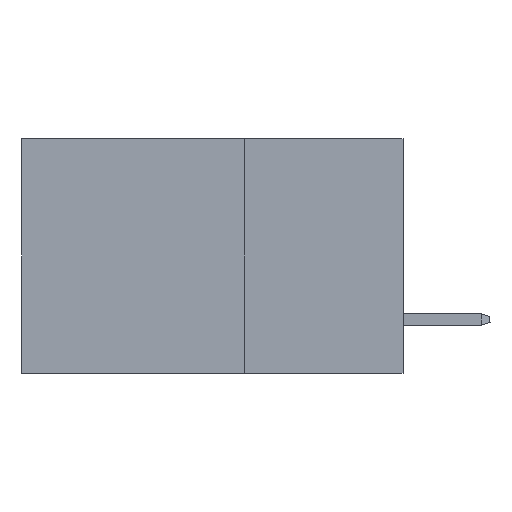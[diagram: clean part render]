
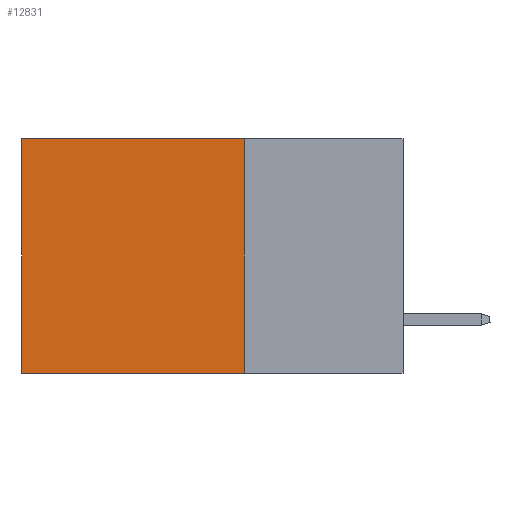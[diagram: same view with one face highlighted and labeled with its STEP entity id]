
A CAD part, left-side view. The second image highlights one B-rep face of the part: STEP entity #12831.
In plain terms, the highlighted planar face has unit normal (-1, 0, 0).
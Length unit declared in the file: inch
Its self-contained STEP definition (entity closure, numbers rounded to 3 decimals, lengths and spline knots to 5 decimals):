
#256 = VERTEX_POINT ( 'NONE', #8918 ) ;
#1142 = CARTESIAN_POINT ( 'NONE',  ( 0.2875, 0.25, -0.37 ) ) ;
#1535 = CARTESIAN_POINT ( 'NONE',  ( 0.2875, 0.25, 0. ) ) ;
#1874 = LINE ( 'NONE', #1535, #11847 ) ;
#2513 = CARTESIAN_POINT ( 'NONE',  ( 0.2875, 0.25, 0. ) ) ;
#3116 = EDGE_CURVE ( 'NONE', #13336, #14258, #14459, .T. ) ;
#3217 = VERTEX_POINT ( 'NONE', #13743 ) ;
#3584 = ORIENTED_EDGE ( 'NONE', *, *, #3116, .F. ) ;
#3779 = CARTESIAN_POINT ( 'NONE',  ( 0.2875, 0.25, 0. ) ) ;
#4141 = CARTESIAN_POINT ( 'NONE',  ( 0.2875, 0.6, 0. ) ) ;
#4988 = VECTOR ( 'NONE', #9345, 39.37008 ) ;
#6195 = DIRECTION ( 'NONE',  ( 0., 1., 0. ) ) ;
#7062 = EDGE_CURVE ( 'NONE', #3217, #14258, #15848, .T. ) ;
#7212 = ORIENTED_EDGE ( 'NONE', *, *, #7062, .T. ) ;
#8063 = EDGE_CURVE ( 'NONE', #256, #3217, #9187, .T. ) ;
#8296 = EDGE_LOOP ( 'NONE', ( #7212, #3584, #14886, #15418 ) ) ;
#8822 = FACE_OUTER_BOUND ( 'NONE', #8296, .T. ) ;
#8918 = CARTESIAN_POINT ( 'NONE',  ( 0.2875, 0.25, 0. ) ) ;
#9187 = LINE ( 'NONE', #2513, #16423 ) ;
#9327 = EDGE_CURVE ( 'NONE', #256, #13336, #1874, .T. ) ;
#9345 = DIRECTION ( 'NONE',  ( 0., 0., -1. ) ) ;
#9765 = CARTESIAN_POINT ( 'NONE',  ( 0.2875, 0.6, -0.37 ) ) ;
#10184 = DIRECTION ( 'NONE',  ( 1., 0., 0. ) ) ;
#11100 = CARTESIAN_POINT ( 'NONE',  ( 0.2875, 0.25, -0.37 ) ) ;
#11428 = VECTOR ( 'NONE', #15500, 39.37008 ) ;
#11847 = VECTOR ( 'NONE', #12195, 39.37008 ) ;
#12195 = DIRECTION ( 'NONE',  ( 0., 0., -1. ) ) ;
#12831 = ADVANCED_FACE ( 'NONE', ( #8822 ), #16748, .F. ) ;
#13008 = AXIS2_PLACEMENT_3D ( 'NONE', #3779, #10184, #16655 ) ;
#13336 = VERTEX_POINT ( 'NONE', #11100 ) ;
#13743 = CARTESIAN_POINT ( 'NONE',  ( 0.2875, 0.6, 0. ) ) ;
#14258 = VERTEX_POINT ( 'NONE', #9765 ) ;
#14459 = LINE ( 'NONE', #1142, #11428 ) ;
#14886 = ORIENTED_EDGE ( 'NONE', *, *, #9327, .F. ) ;
#15418 = ORIENTED_EDGE ( 'NONE', *, *, #8063, .T. ) ;
#15500 = DIRECTION ( 'NONE',  ( 0., 1., 0. ) ) ;
#15848 = LINE ( 'NONE', #4141, #4988 ) ;
#16423 = VECTOR ( 'NONE', #6195, 39.37008 ) ;
#16655 = DIRECTION ( 'NONE',  ( 0., 0., -1. ) ) ;
#16748 = PLANE ( 'NONE',  #13008 ) ;
